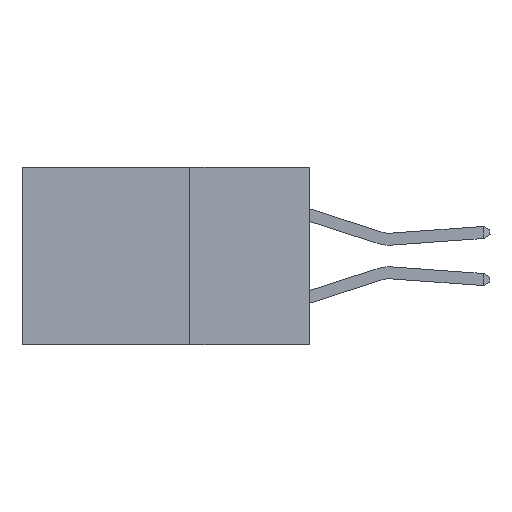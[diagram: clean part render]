
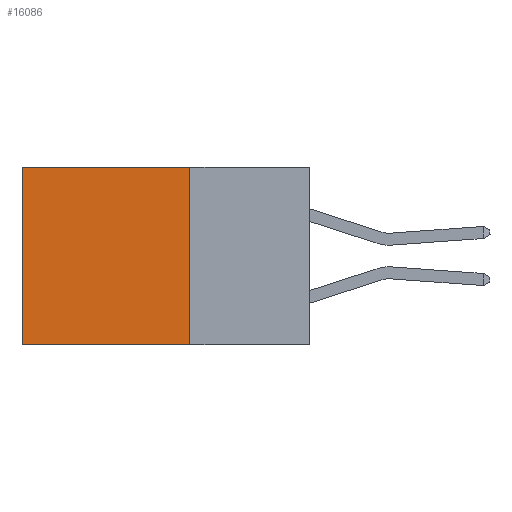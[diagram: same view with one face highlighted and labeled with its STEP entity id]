
A CAD part, left-side view. The second image highlights one B-rep face of the part: STEP entity #16086.
In plain terms, the highlighted planar face has unit normal (-1, 0, 0).
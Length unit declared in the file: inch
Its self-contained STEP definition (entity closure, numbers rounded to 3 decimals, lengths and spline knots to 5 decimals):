
#578 = AXIS2_PLACEMENT_3D ( 'NONE', #15299, #11495, #3574 ) ;
#1595 = CARTESIAN_POINT ( 'NONE',  ( 0.2615, 0.25, -0.37 ) ) ;
#1982 = ORIENTED_EDGE ( 'NONE', *, *, #10373, .T. ) ;
#2035 = DIRECTION ( 'NONE',  ( 0., 1., 0. ) ) ;
#2147 = LINE ( 'NONE', #12520, #14914 ) ;
#2196 = PLANE ( 'NONE',  #578 ) ;
#2224 = CARTESIAN_POINT ( 'NONE',  ( 0.2615, 0.25, 0. ) ) ;
#3574 = DIRECTION ( 'NONE',  ( 0., 0., -1. ) ) ;
#3611 = EDGE_CURVE ( 'NONE', #7002, #15801, #4661, .T. ) ;
#4661 = LINE ( 'NONE', #7895, #11659 ) ;
#6300 = FACE_OUTER_BOUND ( 'NONE', #16390, .T. ) ;
#7002 = VERTEX_POINT ( 'NONE', #14637 ) ;
#7537 = EDGE_CURVE ( 'NONE', #7002, #12312, #7567, .T. ) ;
#7567 = LINE ( 'NONE', #2224, #14055 ) ;
#7895 = CARTESIAN_POINT ( 'NONE',  ( 0.2615, 0.25, -0.37 ) ) ;
#7908 = DIRECTION ( 'NONE',  ( 0., 0., -1. ) ) ;
#8231 = ORIENTED_EDGE ( 'NONE', *, *, #12444, .F. ) ;
#10373 = EDGE_CURVE ( 'NONE', #12312, #10612, #13783, .T. ) ;
#10612 = VERTEX_POINT ( 'NONE', #10682 ) ;
#10682 = CARTESIAN_POINT ( 'NONE',  ( 0.2615, 0.6, -0.37 ) ) ;
#11495 = DIRECTION ( 'NONE',  ( 1., 0., 0. ) ) ;
#11659 = VECTOR ( 'NONE', #7908, 39.37008 ) ;
#12312 = VERTEX_POINT ( 'NONE', #13322 ) ;
#12424 = DIRECTION ( 'NONE',  ( 0., 1., 0. ) ) ;
#12444 = EDGE_CURVE ( 'NONE', #15801, #10612, #2147, .T. ) ;
#12520 = CARTESIAN_POINT ( 'NONE',  ( 0.2615, 0.25, -0.37 ) ) ;
#12964 = VECTOR ( 'NONE', #15246, 39.37008 ) ;
#13203 = ORIENTED_EDGE ( 'NONE', *, *, #7537, .T. ) ;
#13322 = CARTESIAN_POINT ( 'NONE',  ( 0.2615, 0.6, 0. ) ) ;
#13783 = LINE ( 'NONE', #15718, #12964 ) ;
#14055 = VECTOR ( 'NONE', #2035, 39.37008 ) ;
#14637 = CARTESIAN_POINT ( 'NONE',  ( 0.2615, 0.25, 0. ) ) ;
#14914 = VECTOR ( 'NONE', #12424, 39.37008 ) ;
#15246 = DIRECTION ( 'NONE',  ( 0., 0., -1. ) ) ;
#15299 = CARTESIAN_POINT ( 'NONE',  ( 0.2615, 0.25, -0.37 ) ) ;
#15718 = CARTESIAN_POINT ( 'NONE',  ( 0.2615, 0.6, -0.37 ) ) ;
#15801 = VERTEX_POINT ( 'NONE', #1595 ) ;
#16086 = ADVANCED_FACE ( 'NONE', ( #6300 ), #2196, .F. ) ;
#16390 = EDGE_LOOP ( 'NONE', ( #1982, #8231, #16872, #13203 ) ) ;
#16872 = ORIENTED_EDGE ( 'NONE', *, *, #3611, .F. ) ;
